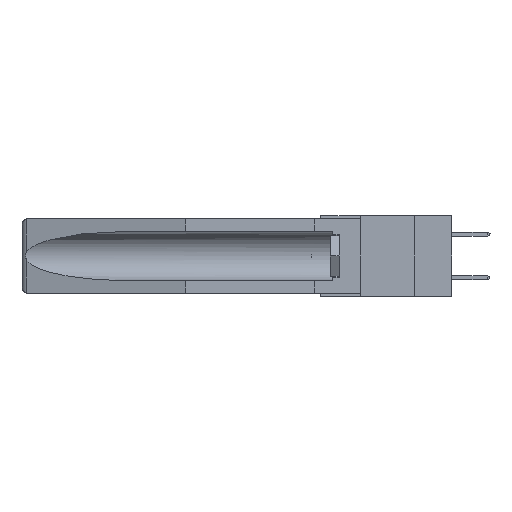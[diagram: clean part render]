
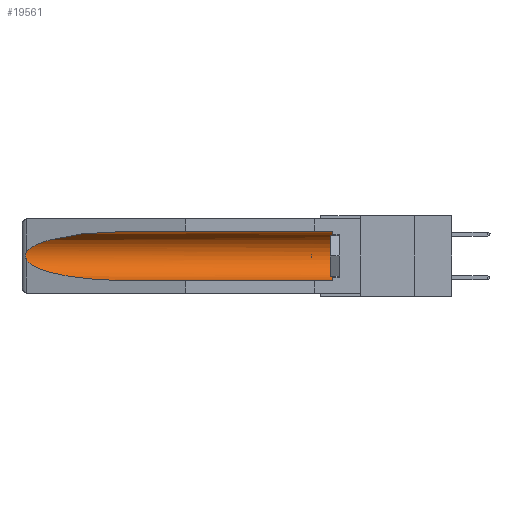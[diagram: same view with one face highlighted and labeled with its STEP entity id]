
A CAD part, left-side view. The second image highlights one B-rep face of the part: STEP entity #19561.
In plain terms, the highlighted cylindrical face has radius 2.857 mm (diameter 5.715 mm), a partial arc.
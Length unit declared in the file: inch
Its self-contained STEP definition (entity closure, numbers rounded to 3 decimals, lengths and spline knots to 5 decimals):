
#287 = CARTESIAN_POINT ( 'NONE',  ( 0.155, 1.07973, -0.284 ) ) ;
#517 = EDGE_LOOP ( 'NONE', ( #4273, #18210, #18742, #9327, #14388, #33437 ) ) ;
#1925 = CARTESIAN_POINT ( 'NONE',  ( 0.155, 1.07973, -0.284 ) ) ;
#2431 = CARTESIAN_POINT ( 'NONE',  ( 0.155, 0.126, -0.284 ) ) ;
#2855 = VERTEX_POINT ( 'NONE', #12767 ) ;
#3803 = VECTOR ( 'NONE', #4583, 39.37008 ) ;
#4273 = ORIENTED_EDGE ( 'NONE', *, *, #9489, .T. ) ;
#4536 = CARTESIAN_POINT ( 'NONE',  ( 0.155, -0.30754, -0.1715 ) ) ;
#4583 = DIRECTION ( 'NONE',  ( 0., 1., 0. ) ) ;
#4644 = CARTESIAN_POINT ( 'NONE',  ( 0.2673, 1.53269, -0.17917 ) ) ;
#4807 = CARTESIAN_POINT ( 'NONE',  ( 0.21114, 1.30732, -0.059 ) ) ;
#5073 = CARTESIAN_POINT ( 'NONE',  ( 0.155, 0.126, -0.1715 ) ) ;
#5558 = CARTESIAN_POINT ( 'NONE',  ( 0.21114, 1.30732, -0.284 ) ) ;
#5654 = AXIS2_PLACEMENT_3D ( 'NONE', #4536, #18810, #23913 ) ;
#6295 = DIRECTION ( 'NONE',  ( 0., 1., 0. ) ) ;
#6511 = CARTESIAN_POINT ( 'NONE',  ( 0.155, -0.30754, -0.284 ) ) ;
#7308 =( BOUNDED_CURVE ( )  B_SPLINE_CURVE ( 3, ( #10492, #4807, #10376, #7822 ),
 .UNSPECIFIED., .F., .F. ) 
 B_SPLINE_CURVE_WITH_KNOTS ( ( 4, 4 ),
 ( 4.71239, 6.08839 ),
 .UNSPECIFIED. ) 
 CURVE ( )  GEOMETRIC_REPRESENTATION_ITEM ( )  RATIONAL_B_SPLINE_CURVE ( ( 1., 0.848, 0.848, 1. ) ) 
 REPRESENTATION_ITEM ( '' )  );
#7747 = VECTOR ( 'NONE', #6295, 39.37008 ) ;
#7822 = CARTESIAN_POINT ( 'NONE',  ( 0.26537, 1.52718, -0.14972 ) ) ;
#8104 = CARTESIAN_POINT ( 'NONE',  ( 0.26537, 1.52718, -0.19328 ) ) ;
#9327 = ORIENTED_EDGE ( 'NONE', *, *, #23773, .F. ) ;
#9489 = EDGE_CURVE ( 'NONE', #2855, #24045, #7308, .T. ) ;
#9762 = VERTEX_POINT ( 'NONE', #25849 ) ;
#10376 = CARTESIAN_POINT ( 'NONE',  ( 0.25451, 1.48313, -0.09465 ) ) ;
#10492 = CARTESIAN_POINT ( 'NONE',  ( 0.155, 1.07973, -0.059 ) ) ;
#12387 =( BOUNDED_CURVE ( )  B_SPLINE_CURVE ( 3, ( #8104, #13681, #5558, #287 ),
 .UNSPECIFIED., .F., .F. ) 
 B_SPLINE_CURVE_WITH_KNOTS ( ( 4, 4 ),
 ( 0.1948, 1.5708 ),
 .UNSPECIFIED. ) 
 CURVE ( )  GEOMETRIC_REPRESENTATION_ITEM ( )  RATIONAL_B_SPLINE_CURVE ( ( 1., 0.848, 0.848, 1. ) ) 
 REPRESENTATION_ITEM ( '' )  );
#12645 = CARTESIAN_POINT ( 'NONE',  ( 0.2673, 1.5327, -0.16383 ) ) ;
#12767 = CARTESIAN_POINT ( 'NONE',  ( 0.155, 1.07973, -0.059 ) ) ;
#13681 = CARTESIAN_POINT ( 'NONE',  ( 0.25451, 1.48313, -0.24835 ) ) ;
#14388 = ORIENTED_EDGE ( 'NONE', *, *, #14965, .T. ) ;
#14965 = EDGE_CURVE ( 'NONE', #33219, #9762, #34145, .T. ) ;
#15563 = AXIS2_PLACEMENT_3D ( 'NONE', #5073, #24084, #32486 ) ;
#15587 = CARTESIAN_POINT ( 'NONE',  ( 0.155, -0.30754, -0.059 ) ) ;
#15772 = CARTESIAN_POINT ( 'NONE',  ( 0.26597, 1.52961, -0.15275 ) ) ;
#18082 = CARTESIAN_POINT ( 'NONE',  ( 0.2675, 1.53308, -0.17534 ) ) ;
#18193 = CARTESIAN_POINT ( 'NONE',  ( 0.26537, 1.52718, -0.19328 ) ) ;
#18210 = ORIENTED_EDGE ( 'NONE', *, *, #26063, .T. ) ;
#18322 = CARTESIAN_POINT ( 'NONE',  ( 0.2675, 1.53308, -0.16763 ) ) ;
#18742 = ORIENTED_EDGE ( 'NONE', *, *, #29542, .T. ) ;
#18810 = DIRECTION ( 'NONE',  ( 0., 1., 0. ) ) ;
#19561 = ADVANCED_FACE ( 'NONE', ( #35433 ), #23695, .F. ) ;
#21517 = B_SPLINE_CURVE_WITH_KNOTS ( 'NONE', 3,
 ( #26710, #15772, #29360, #12645, #18322, #18082, #4644, #32066, #35092, #18193 ),
 .UNSPECIFIED., .F., .F.,
 ( 4, 2, 2, 2, 4 ),
 ( 0., 0.00029, 0.00058, 0.00087, 0.00117 ),
 .UNSPECIFIED. ) ;
#22305 = VERTEX_POINT ( 'NONE', #1925 ) ;
#23282 = LINE ( 'NONE', #15587, #3803 ) ;
#23695 = CYLINDRICAL_SURFACE ( 'NONE', #5654, 0.1125 ) ;
#23773 = EDGE_CURVE ( 'NONE', #33219, #22305, #28577, .T. ) ;
#23913 = DIRECTION ( 'NONE',  ( 0., 0., 1. ) ) ;
#24045 = VERTEX_POINT ( 'NONE', #27097 ) ;
#24084 = DIRECTION ( 'NONE',  ( 0., -1., 0. ) ) ;
#24676 = EDGE_CURVE ( 'NONE', #9762, #2855, #23282, .T. ) ;
#25849 = CARTESIAN_POINT ( 'NONE',  ( 0.155, 0.126, -0.059 ) ) ;
#26063 = EDGE_CURVE ( 'NONE', #24045, #29963, #21517, .T. ) ;
#26710 = CARTESIAN_POINT ( 'NONE',  ( 0.26537, 1.52718, -0.14972 ) ) ;
#27097 = CARTESIAN_POINT ( 'NONE',  ( 0.26537, 1.52718, -0.14972 ) ) ;
#28577 = LINE ( 'NONE', #6511, #7747 ) ;
#29360 = CARTESIAN_POINT ( 'NONE',  ( 0.26654, 1.53092, -0.15636 ) ) ;
#29542 = EDGE_CURVE ( 'NONE', #29963, #22305, #12387, .T. ) ;
#29963 = VERTEX_POINT ( 'NONE', #35569 ) ;
#32066 = CARTESIAN_POINT ( 'NONE',  ( 0.26655, 1.53094, -0.18657 ) ) ;
#32486 = DIRECTION ( 'NONE',  ( 0., 0., 1. ) ) ;
#33219 = VERTEX_POINT ( 'NONE', #2431 ) ;
#33437 = ORIENTED_EDGE ( 'NONE', *, *, #24676, .T. ) ;
#34145 = CIRCLE ( 'NONE', #15563, 0.1125 ) ;
#35092 = CARTESIAN_POINT ( 'NONE',  ( 0.26597, 1.5296, -0.19026 ) ) ;
#35433 = FACE_OUTER_BOUND ( 'NONE', #517, .T. ) ;
#35569 = CARTESIAN_POINT ( 'NONE',  ( 0.26537, 1.52718, -0.19328 ) ) ;
